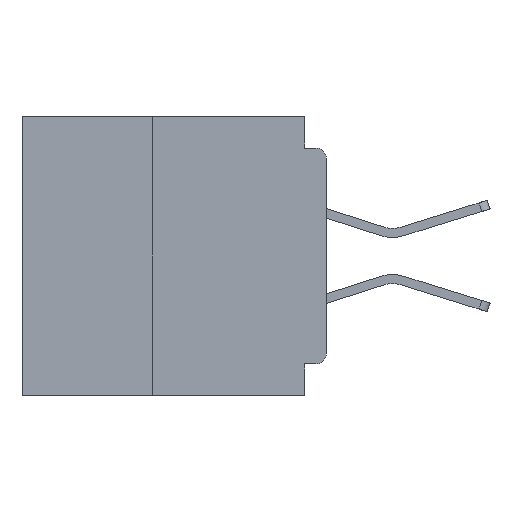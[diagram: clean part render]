
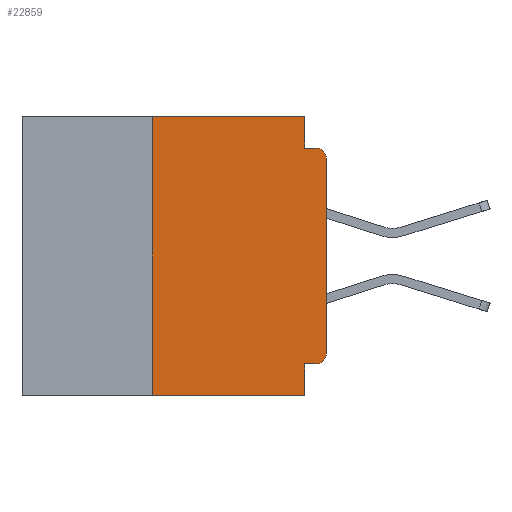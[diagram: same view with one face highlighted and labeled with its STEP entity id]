
A CAD part, left-side view. The second image highlights one B-rep face of the part: STEP entity #22859.
In plain terms, the highlighted planar face has unit normal (-1, 0, 0).
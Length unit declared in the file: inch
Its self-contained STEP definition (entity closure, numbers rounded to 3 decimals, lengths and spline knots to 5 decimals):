
#1565 = CARTESIAN_POINT ( 'NONE',  ( 0., 0.437, 0. ) ) ;
#4243 = ORIENTED_EDGE ( 'NONE', *, *, #46252, .T. ) ;
#5817 = EDGE_CURVE ( 'NONE', #20028, #31972, #25935, .T. ) ;
#6647 = EDGE_CURVE ( 'NONE', #17509, #31486, #27281, .T. ) ;
#6950 = CARTESIAN_POINT ( 'NONE',  ( 0., 0.031, -0.4 ) ) ;
#6984 = VERTEX_POINT ( 'NONE', #17371 ) ;
#7278 = DIRECTION ( 'NONE',  ( 0., 1., 0. ) ) ;
#8045 = CARTESIAN_POINT ( 'NONE',  ( 0., 0.437, 0. ) ) ;
#8374 = VECTOR ( 'NONE', #12752, 39.37008 ) ;
#8661 = AXIS2_PLACEMENT_3D ( 'NONE', #38769, #10637, #43442 ) ;
#9947 = VECTOR ( 'NONE', #50907, 39.37008 ) ;
#10637 = DIRECTION ( 'NONE',  ( -1., 0., 0. ) ) ;
#11345 = AXIS2_PLACEMENT_3D ( 'NONE', #1565, #25322, #57901 ) ;
#11677 = DIRECTION ( 'NONE',  ( 0., 0., -1. ) ) ;
#12518 = LINE ( 'NONE', #30121, #17154 ) ;
#12752 = DIRECTION ( 'NONE',  ( 0., -1., 0. ) ) ;
#13480 = VERTEX_POINT ( 'NONE', #40183 ) ;
#13640 = VECTOR ( 'NONE', #11677, 39.37008 ) ;
#13909 = VECTOR ( 'NONE', #42890, 39.37008 ) ;
#14545 = ORIENTED_EDGE ( 'NONE', *, *, #15832, .F. ) ;
#15832 = EDGE_CURVE ( 'NONE', #6984, #31972, #50957, .T. ) ;
#15840 = ORIENTED_EDGE ( 'NONE', *, *, #45885, .F. ) ;
#16122 = EDGE_CURVE ( 'NONE', #55604, #31486, #59661, .T. ) ;
#16456 = CARTESIAN_POINT ( 'NONE',  ( 0., 0., -0.34 ) ) ;
#16511 = CARTESIAN_POINT ( 'NONE',  ( 0., 0., -0.355 ) ) ;
#16531 = VECTOR ( 'NONE', #55008, 39.37008 ) ;
#17154 = VECTOR ( 'NONE', #39516, 39.37008 ) ;
#17371 = CARTESIAN_POINT ( 'NONE',  ( 0., 0.031, -0.355 ) ) ;
#17509 = VERTEX_POINT ( 'NONE', #40495 ) ;
#19658 = EDGE_CURVE ( 'NONE', #20028, #26372, #19830, .T. ) ;
#19685 = CARTESIAN_POINT ( 'NONE',  ( 0., 0.015, -0.06 ) ) ;
#19830 = LINE ( 'NONE', #51990, #13909 ) ;
#20028 = VERTEX_POINT ( 'NONE', #46895 ) ;
#22048 = CARTESIAN_POINT ( 'NONE',  ( 0., 0.437, -0.4 ) ) ;
#22251 = DIRECTION ( 'NONE',  ( 0., -1., 0. ) ) ;
#22414 = CARTESIAN_POINT ( 'NONE',  ( 0., 0.031, 0. ) ) ;
#22859 = ADVANCED_FACE ( 'NONE', ( #30547 ), #53172, .F. ) ;
#23001 = CARTESIAN_POINT ( 'NONE',  ( 0., 0., -0.045 ) ) ;
#24438 = DIRECTION ( 'NONE',  ( 0., 0., -1. ) ) ;
#25300 = CIRCLE ( 'NONE', #8661, 0.015 ) ;
#25322 = DIRECTION ( 'NONE',  ( 1., 0., 0. ) ) ;
#25341 = CARTESIAN_POINT ( 'NONE',  ( 0., 0.015, -0.045 ) ) ;
#25583 = ORIENTED_EDGE ( 'NONE', *, *, #5817, .T. ) ;
#25935 = LINE ( 'NONE', #22048, #35431 ) ;
#26184 = VECTOR ( 'NONE', #7278, 39.37008 ) ;
#26305 = ORIENTED_EDGE ( 'NONE', *, *, #19658, .F. ) ;
#26372 = VERTEX_POINT ( 'NONE', #57586 ) ;
#27281 = CIRCLE ( 'NONE', #38020, 0.015 ) ;
#30121 = CARTESIAN_POINT ( 'NONE',  ( 0., 0., 0. ) ) ;
#30547 = FACE_OUTER_BOUND ( 'NONE', #34838, .T. ) ;
#31486 = VERTEX_POINT ( 'NONE', #25341 ) ;
#31909 = ORIENTED_EDGE ( 'NONE', *, *, #32324, .T. ) ;
#31972 = VERTEX_POINT ( 'NONE', #41590 ) ;
#32324 = EDGE_CURVE ( 'NONE', #32878, #17509, #12518, .T. ) ;
#32878 = VERTEX_POINT ( 'NONE', #16456 ) ;
#34366 = CARTESIAN_POINT ( 'NONE',  ( 0., 0.031, -0.045 ) ) ;
#34838 = EDGE_LOOP ( 'NONE', ( #31909, #53011, #58248, #38730, #15840, #26305, #25583, #14545, #38831, #4243 ) ) ;
#35431 = VECTOR ( 'NONE', #22251, 39.37008 ) ;
#36040 = EDGE_CURVE ( 'NONE', #13480, #55604, #53816, .T. ) ;
#38020 = AXIS2_PLACEMENT_3D ( 'NONE', #19685, #52311, #24438 ) ;
#38599 = LINE ( 'NONE', #16511, #26184 ) ;
#38730 = ORIENTED_EDGE ( 'NONE', *, *, #36040, .F. ) ;
#38769 = CARTESIAN_POINT ( 'NONE',  ( 0., 0.015, -0.34 ) ) ;
#38831 = ORIENTED_EDGE ( 'NONE', *, *, #50332, .F. ) ;
#39516 = DIRECTION ( 'NONE',  ( 0., 0., 1. ) ) ;
#40183 = CARTESIAN_POINT ( 'NONE',  ( 0., 0.031, 0. ) ) ;
#40495 = CARTESIAN_POINT ( 'NONE',  ( 0., 0., -0.06 ) ) ;
#41590 = CARTESIAN_POINT ( 'NONE',  ( 0., 0.031, -0.4 ) ) ;
#42890 = DIRECTION ( 'NONE',  ( 0., 0., 1. ) ) ;
#43442 = DIRECTION ( 'NONE',  ( 0., 0., -1. ) ) ;
#45885 = EDGE_CURVE ( 'NONE', #26372, #13480, #59553, .T. ) ;
#46252 = EDGE_CURVE ( 'NONE', #54487, #32878, #25300, .T. ) ;
#46895 = CARTESIAN_POINT ( 'NONE',  ( 0., 0.25, -0.4 ) ) ;
#50332 = EDGE_CURVE ( 'NONE', #54487, #6984, #38599, .T. ) ;
#50907 = DIRECTION ( 'NONE',  ( 0., -1., 0. ) ) ;
#50957 = LINE ( 'NONE', #6950, #13640 ) ;
#51990 = CARTESIAN_POINT ( 'NONE',  ( 0., 0.25, -0.4 ) ) ;
#52311 = DIRECTION ( 'NONE',  ( -1., 0., 0. ) ) ;
#53011 = ORIENTED_EDGE ( 'NONE', *, *, #6647, .T. ) ;
#53172 = PLANE ( 'NONE',  #11345 ) ;
#53816 = LINE ( 'NONE', #22414, #16531 ) ;
#54487 = VERTEX_POINT ( 'NONE', #54933 ) ;
#54933 = CARTESIAN_POINT ( 'NONE',  ( 0., 0.015, -0.355 ) ) ;
#55008 = DIRECTION ( 'NONE',  ( 0., 0., -1. ) ) ;
#55604 = VERTEX_POINT ( 'NONE', #34366 ) ;
#57586 = CARTESIAN_POINT ( 'NONE',  ( 0., 0.25, 0. ) ) ;
#57901 = DIRECTION ( 'NONE',  ( 0., 0., -1. ) ) ;
#58248 = ORIENTED_EDGE ( 'NONE', *, *, #16122, .F. ) ;
#59553 = LINE ( 'NONE', #8045, #8374 ) ;
#59661 = LINE ( 'NONE', #23001, #9947 ) ;
